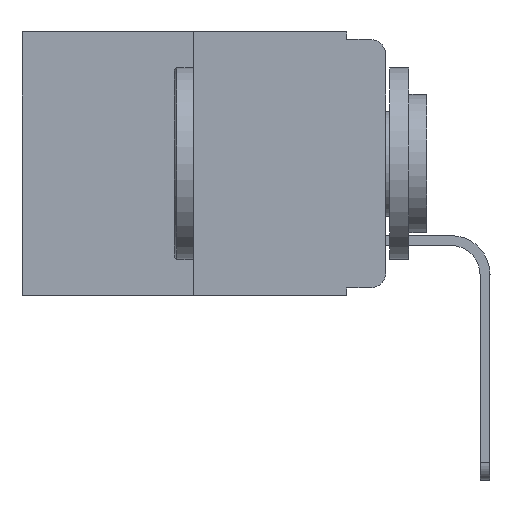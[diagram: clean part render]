
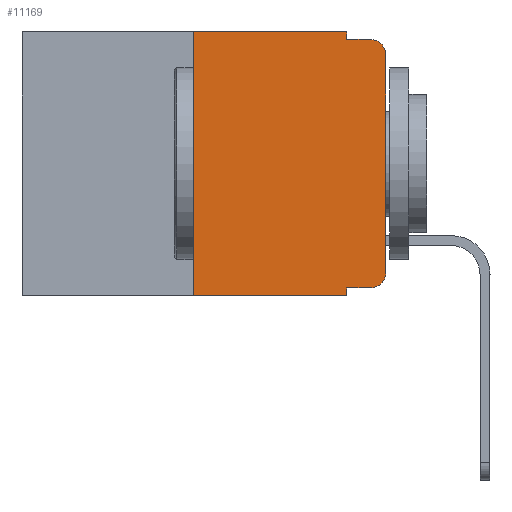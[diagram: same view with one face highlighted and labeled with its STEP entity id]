
A CAD part, left-side view. The second image highlights one B-rep face of the part: STEP entity #11169.
In plain terms, the highlighted planar face has unit normal (-1, 0, 0).
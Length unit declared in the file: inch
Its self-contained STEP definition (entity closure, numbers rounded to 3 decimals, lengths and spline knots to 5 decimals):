
#87 = ORIENTED_EDGE ( 'NONE', *, *, #14439, .T. ) ;
#184 = ORIENTED_EDGE ( 'NONE', *, *, #22021, .T. ) ;
#644 = ORIENTED_EDGE ( 'NONE', *, *, #19900, .F. ) ;
#858 = DIRECTION ( 'NONE',  ( -1., 0., 0. ) ) ;
#2122 = EDGE_CURVE ( 'NONE', #14078, #15694, #12216, .T. ) ;
#2179 = VECTOR ( 'NONE', #10390, 39.37008 ) ;
#2301 = DIRECTION ( 'NONE',  ( 0., 0., 1. ) ) ;
#2520 = VERTEX_POINT ( 'NONE', #3877 ) ;
#2562 = CARTESIAN_POINT ( 'NONE',  ( 0., 0.051, 0. ) ) ;
#2585 = DIRECTION ( 'NONE',  ( 0., 0., -1. ) ) ;
#2664 = CARTESIAN_POINT ( 'NONE',  ( 0., 0.02, -0.03 ) ) ;
#2931 = DIRECTION ( 'NONE',  ( 0., -1., 0. ) ) ;
#3410 = VECTOR ( 'NONE', #17596, 39.37008 ) ;
#3816 = VERTEX_POINT ( 'NONE', #11127 ) ;
#3877 = CARTESIAN_POINT ( 'NONE',  ( 0., 0.051, -0.343 ) ) ;
#3890 = DIRECTION ( 'NONE',  ( 0., 0., -1. ) ) ;
#4190 = PLANE ( 'NONE',  #10223 ) ;
#4517 = LINE ( 'NONE', #14853, #16201 ) ;
#4720 = CARTESIAN_POINT ( 'NONE',  ( 0., 0.25, 0. ) ) ;
#4839 = EDGE_CURVE ( 'NONE', #14078, #2520, #11265, .T. ) ;
#4885 = EDGE_CURVE ( 'NONE', #6438, #5576, #4517, .T. ) ;
#4955 = CIRCLE ( 'NONE', #19221, 0.02 ) ;
#5474 = VERTEX_POINT ( 'NONE', #19256 ) ;
#5576 = VERTEX_POINT ( 'NONE', #8768 ) ;
#6260 = VECTOR ( 'NONE', #6765, 39.37008 ) ;
#6438 = VERTEX_POINT ( 'NONE', #20985 ) ;
#6450 = VECTOR ( 'NONE', #11338, 39.37008 ) ;
#6589 = DIRECTION ( 'NONE',  ( 0., 0., -1. ) ) ;
#6765 = DIRECTION ( 'NONE',  ( 0., 0., -1. ) ) ;
#7589 = FACE_OUTER_BOUND ( 'NONE', #17123, .T. ) ;
#7694 = DIRECTION ( 'NONE',  ( 1., 0., 0. ) ) ;
#8604 = EDGE_CURVE ( 'NONE', #15694, #11222, #16847, .T. ) ;
#8768 = CARTESIAN_POINT ( 'NONE',  ( 0., 0.02, -0.333 ) ) ;
#8949 = CIRCLE ( 'NONE', #20115, 0.02 ) ;
#9433 = ORIENTED_EDGE ( 'NONE', *, *, #20539, .T. ) ;
#9441 = DIRECTION ( 'NONE',  ( 0., 0., -1. ) ) ;
#9569 = CARTESIAN_POINT ( 'NONE',  ( 0., 0.25, -0.343 ) ) ;
#9919 = CARTESIAN_POINT ( 'NONE',  ( 0., 0.051, 0. ) ) ;
#10223 = AXIS2_PLACEMENT_3D ( 'NONE', #16330, #7694, #3890 ) ;
#10390 = DIRECTION ( 'NONE',  ( 0., 0., 1. ) ) ;
#10629 = LINE ( 'NONE', #17233, #2179 ) ;
#10983 = ORIENTED_EDGE ( 'NONE', *, *, #2122, .F. ) ;
#11127 = CARTESIAN_POINT ( 'NONE',  ( 0., 0., -0.313 ) ) ;
#11169 = ADVANCED_FACE ( 'NONE', ( #7589 ), #4190, .F. ) ;
#11222 = VERTEX_POINT ( 'NONE', #2562 ) ;
#11265 = LINE ( 'NONE', #11982, #3410 ) ;
#11338 = DIRECTION ( 'NONE',  ( 0., -1., 0. ) ) ;
#11472 = CARTESIAN_POINT ( 'NONE',  ( 0., 0.02, -0.313 ) ) ;
#11783 = ORIENTED_EDGE ( 'NONE', *, *, #4839, .T. ) ;
#11921 = EDGE_CURVE ( 'NONE', #19429, #16851, #19482, .T. ) ;
#11982 = CARTESIAN_POINT ( 'NONE',  ( 0., 0.473, -0.343 ) ) ;
#12216 = LINE ( 'NONE', #21589, #17947 ) ;
#13058 = CARTESIAN_POINT ( 'NONE',  ( 0., 0.02, -0.01 ) ) ;
#13563 = LINE ( 'NONE', #9919, #18482 ) ;
#13854 = ORIENTED_EDGE ( 'NONE', *, *, #11921, .F. ) ;
#14078 = VERTEX_POINT ( 'NONE', #9569 ) ;
#14439 = EDGE_CURVE ( 'NONE', #3816, #5474, #10629, .T. ) ;
#14669 = LINE ( 'NONE', #16999, #6260 ) ;
#14853 = CARTESIAN_POINT ( 'NONE',  ( 0., 0.051, -0.333 ) ) ;
#14952 = CARTESIAN_POINT ( 'NONE',  ( 0., 0.473, 0. ) ) ;
#15694 = VERTEX_POINT ( 'NONE', #4720 ) ;
#16201 = VECTOR ( 'NONE', #16750, 39.37008 ) ;
#16330 = CARTESIAN_POINT ( 'NONE',  ( 0., 0.473, 0. ) ) ;
#16377 = ORIENTED_EDGE ( 'NONE', *, *, #4885, .T. ) ;
#16750 = DIRECTION ( 'NONE',  ( 0., -1., 0. ) ) ;
#16847 = LINE ( 'NONE', #14952, #21729 ) ;
#16851 = VERTEX_POINT ( 'NONE', #13058 ) ;
#16999 = CARTESIAN_POINT ( 'NONE',  ( 0., 0.051, 0. ) ) ;
#17123 = EDGE_LOOP ( 'NONE', ( #87, #184, #13854, #644, #21272, #10983, #11783, #19000, #16377, #9433 ) ) ;
#17233 = CARTESIAN_POINT ( 'NONE',  ( 0., 0., 0. ) ) ;
#17596 = DIRECTION ( 'NONE',  ( 0., -1., 0. ) ) ;
#17947 = VECTOR ( 'NONE', #2301, 39.37008 ) ;
#18109 = DIRECTION ( 'NONE',  ( -1., 0., 0. ) ) ;
#18482 = VECTOR ( 'NONE', #6589, 39.37008 ) ;
#19000 = ORIENTED_EDGE ( 'NONE', *, *, #19329, .F. ) ;
#19221 = AXIS2_PLACEMENT_3D ( 'NONE', #11472, #858, #9441 ) ;
#19256 = CARTESIAN_POINT ( 'NONE',  ( 0., 0., -0.03 ) ) ;
#19329 = EDGE_CURVE ( 'NONE', #6438, #2520, #14669, .T. ) ;
#19429 = VERTEX_POINT ( 'NONE', #20494 ) ;
#19482 = LINE ( 'NONE', #21750, #6450 ) ;
#19900 = EDGE_CURVE ( 'NONE', #11222, #19429, #13563, .T. ) ;
#20115 = AXIS2_PLACEMENT_3D ( 'NONE', #2664, #18109, #2585 ) ;
#20494 = CARTESIAN_POINT ( 'NONE',  ( 0., 0.051, -0.01 ) ) ;
#20539 = EDGE_CURVE ( 'NONE', #5576, #3816, #4955, .T. ) ;
#20985 = CARTESIAN_POINT ( 'NONE',  ( 0., 0.051, -0.333 ) ) ;
#21272 = ORIENTED_EDGE ( 'NONE', *, *, #8604, .F. ) ;
#21589 = CARTESIAN_POINT ( 'NONE',  ( 0., 0.25, 0. ) ) ;
#21729 = VECTOR ( 'NONE', #2931, 39.37008 ) ;
#21750 = CARTESIAN_POINT ( 'NONE',  ( 0., 0.051, -0.01 ) ) ;
#22021 = EDGE_CURVE ( 'NONE', #5474, #16851, #8949, .T. ) ;
